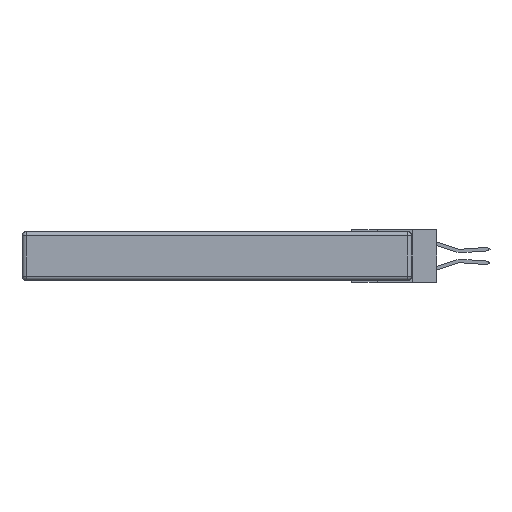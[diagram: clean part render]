
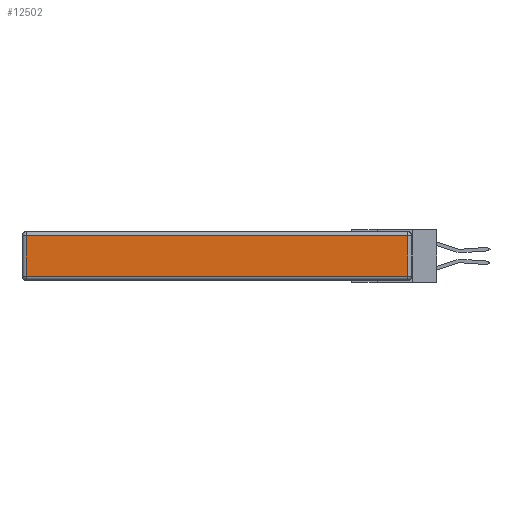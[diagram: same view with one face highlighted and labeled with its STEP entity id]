
A CAD part, left-side view. The second image highlights one B-rep face of the part: STEP entity #12502.
In plain terms, the highlighted planar face has unit normal (-1, 0, 0).
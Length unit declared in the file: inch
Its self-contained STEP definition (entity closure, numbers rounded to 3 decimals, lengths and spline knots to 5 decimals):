
#1808 = ORIENTED_EDGE ( 'NONE', *, *, #4710, .T. ) ;
#2326 = LINE ( 'NONE', #22226, #7468 ) ;
#2450 = AXIS2_PLACEMENT_3D ( 'NONE', #14046, #21413, #12512 ) ;
#4465 = VERTEX_POINT ( 'NONE', #23907 ) ;
#4710 = EDGE_CURVE ( 'NONE', #6498, #17534, #5806, .T. ) ;
#5023 = CARTESIAN_POINT ( 'NONE',  ( 0., 2.72, -0.03 ) ) ;
#5806 = LINE ( 'NONE', #14594, #26082 ) ;
#6498 = VERTEX_POINT ( 'NONE', #13363 ) ;
#7468 = VECTOR ( 'NONE', #8985, 39.37008 ) ;
#7471 = VECTOR ( 'NONE', #9614, 39.37008 ) ;
#7835 = FACE_OUTER_BOUND ( 'NONE', #17180, .T. ) ;
#8101 = DIRECTION ( 'NONE',  ( 0., -1., 0. ) ) ;
#8579 = VECTOR ( 'NONE', #15177, 39.37008 ) ;
#8985 = DIRECTION ( 'NONE',  ( 0., 1., 0. ) ) ;
#9614 = DIRECTION ( 'NONE',  ( 0., 0., 1. ) ) ;
#9852 = LINE ( 'NONE', #20650, #7471 ) ;
#11286 = EDGE_CURVE ( 'NONE', #21807, #6498, #11348, .T. ) ;
#11348 = LINE ( 'NONE', #28343, #8579 ) ;
#12502 = ADVANCED_FACE ( 'NONE', ( #7835 ), #24987, .T. ) ;
#12512 = DIRECTION ( 'NONE',  ( 0., 0., 1. ) ) ;
#13363 = CARTESIAN_POINT ( 'NONE',  ( 0., 2.72, -0.313 ) ) ;
#14046 = CARTESIAN_POINT ( 'NONE',  ( 0., 0., -0.343 ) ) ;
#14551 = ORIENTED_EDGE ( 'NONE', *, *, #11286, .T. ) ;
#14594 = CARTESIAN_POINT ( 'NONE',  ( 0., 0., -0.313 ) ) ;
#15177 = DIRECTION ( 'NONE',  ( 0., 0., -1. ) ) ;
#15539 = ORIENTED_EDGE ( 'NONE', *, *, #25035, .T. ) ;
#17180 = EDGE_LOOP ( 'NONE', ( #1808, #24235, #15539, #14551 ) ) ;
#17534 = VERTEX_POINT ( 'NONE', #23728 ) ;
#17931 = EDGE_CURVE ( 'NONE', #17534, #4465, #9852, .T. ) ;
#20650 = CARTESIAN_POINT ( 'NONE',  ( 0., 0.03, -0.343 ) ) ;
#21413 = DIRECTION ( 'NONE',  ( -1., 0., 0. ) ) ;
#21807 = VERTEX_POINT ( 'NONE', #5023 ) ;
#22226 = CARTESIAN_POINT ( 'NONE',  ( 0., 2.75, -0.03 ) ) ;
#23728 = CARTESIAN_POINT ( 'NONE',  ( 0., 0.03, -0.313 ) ) ;
#23907 = CARTESIAN_POINT ( 'NONE',  ( 0., 0.03, -0.03 ) ) ;
#24235 = ORIENTED_EDGE ( 'NONE', *, *, #17931, .T. ) ;
#24987 = PLANE ( 'NONE',  #2450 ) ;
#25035 = EDGE_CURVE ( 'NONE', #4465, #21807, #2326, .T. ) ;
#26082 = VECTOR ( 'NONE', #8101, 39.37008 ) ;
#28343 = CARTESIAN_POINT ( 'NONE',  ( 0., 2.72, -0.343 ) ) ;
